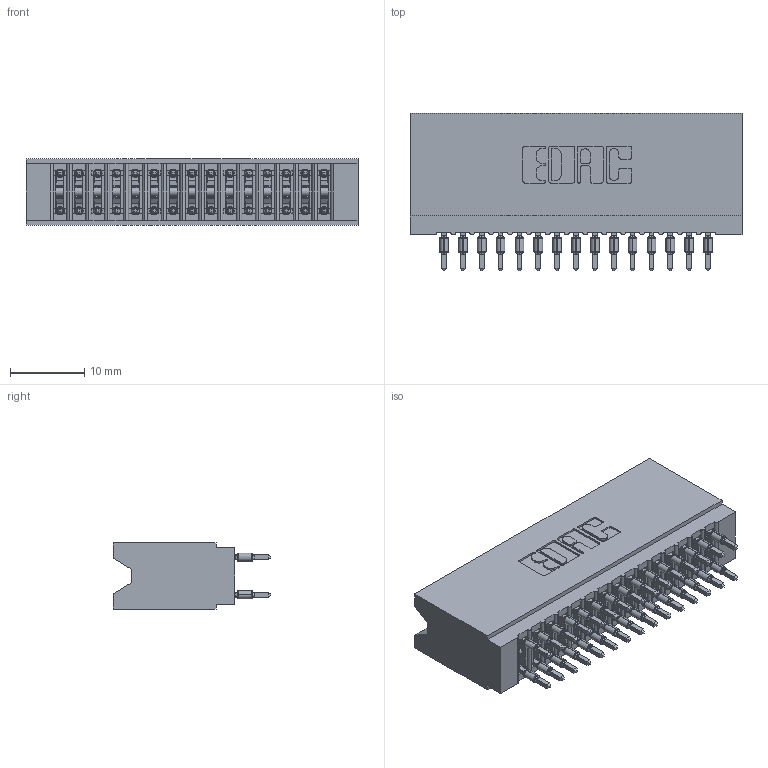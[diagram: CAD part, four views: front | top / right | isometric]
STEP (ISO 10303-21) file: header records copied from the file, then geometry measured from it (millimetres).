
FILE_DESCRIPTION (( 'STEP AP203' ), '1' );
FILE_NAME ('745-030-560-206.STEP', '2020-09-11T20:23:00', ( '' ), ( '' ), 'SwSTEP 2.0', 'SolidWorks 2020', '' );
FILE_SCHEMA (( 'CONFIG_CONTROL_DESIGN' ));
Length unit declared in the file: inch
Products named in the file (3): 745-292-001_560; 745-030-560-206; 745 Part_Insulator Option - 06
Assembly tree (31 placements, depth 2):
  745-030-560-206
    745 Part_Insulator Option - 06
    745-292-001_560  x30
Bounding box: 44.7 x 21.22 x 8.89 mm (x, y, z)
Volume: 4277.6 mm3; surface area: 8571.4 mm2
Topology: 31 solids, 31 shells, 3051 faces, 8345 edges, 5302 vertices
Faces by surface type: plane 1586, cylinder 685, bspline 600, torus 180
Entity records: 29288 total; most frequent: CARTESIAN_POINT 5592, ORIENTED_EDGE 4974, DIRECTION 4373, EDGE_CURVE 2487, LINE 2207, VECTOR 2207, VERTEX_POINT 1590, AXIS2_PLACEMENT_3D 1083
